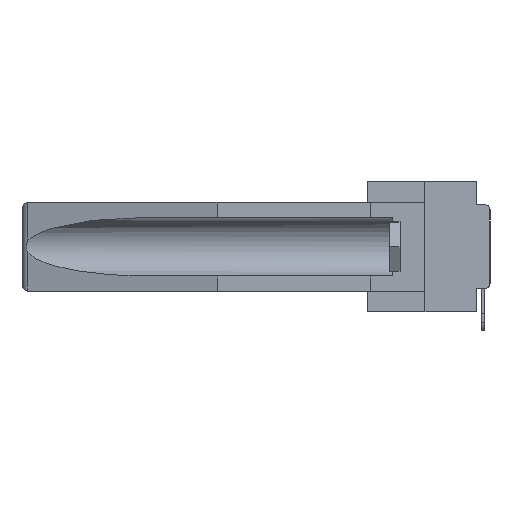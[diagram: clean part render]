
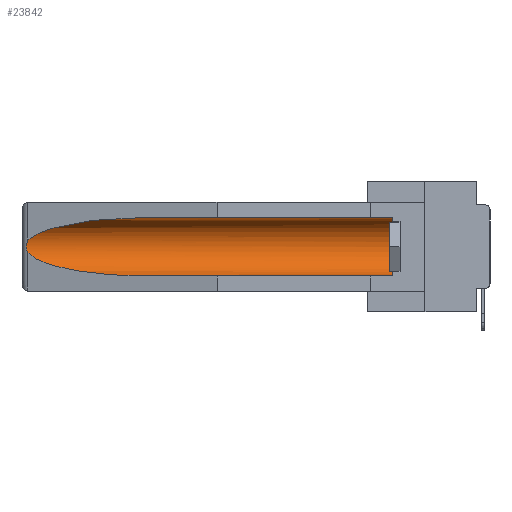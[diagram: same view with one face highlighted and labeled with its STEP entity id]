
A CAD part, left-side view. The second image highlights one B-rep face of the part: STEP entity #23842.
In plain terms, the highlighted cylindrical face has radius 2.857 mm (diameter 5.715 mm), a partial arc.
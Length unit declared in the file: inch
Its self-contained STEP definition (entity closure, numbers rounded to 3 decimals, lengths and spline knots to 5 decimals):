
#638 = ORIENTED_EDGE ( 'NONE', *, *, #23297, .T. ) ;
#746 = CARTESIAN_POINT ( 'NONE',  ( 0.21114, 1.30732, -0.284 ) ) ;
#1210 = EDGE_LOOP ( 'NONE', ( #5220, #638, #20879, #20335, #5488, #31208 ) ) ;
#1312 = DIRECTION ( 'NONE',  ( 0., 0., 1. ) ) ;
#1347 = CARTESIAN_POINT ( 'NONE',  ( 0.2673, 1.5327, -0.16383 ) ) ;
#1713 = EDGE_CURVE ( 'NONE', #22830, #21213, #23108, .T. ) ;
#2689 = EDGE_CURVE ( 'NONE', #28730, #30692, #25787, .T. ) ;
#2841 = VECTOR ( 'NONE', #15297, 39.37008 ) ;
#3569 = DIRECTION ( 'NONE',  ( 0., 1., 0. ) ) ;
#3854 = CYLINDRICAL_SURFACE ( 'NONE', #14177, 0.1125 ) ;
#4030 = CARTESIAN_POINT ( 'NONE',  ( 0.26597, 1.52961, -0.15275 ) ) ;
#4127 = CARTESIAN_POINT ( 'NONE',  ( 0.26537, 1.52718, -0.14972 ) ) ;
#4273 = CARTESIAN_POINT ( 'NONE',  ( 0.21114, 1.30732, -0.059 ) ) ;
#4820 = CARTESIAN_POINT ( 'NONE',  ( 0.155, 1.07973, -0.059 ) ) ;
#4983 = CARTESIAN_POINT ( 'NONE',  ( 0.155, 0.126, -0.284 ) ) ;
#5220 = ORIENTED_EDGE ( 'NONE', *, *, #10701, .T. ) ;
#5488 = ORIENTED_EDGE ( 'NONE', *, *, #2689, .T. ) ;
#5899 = CARTESIAN_POINT ( 'NONE',  ( 0.26537, 1.52718, -0.19328 ) ) ;
#6040 = DIRECTION ( 'NONE',  ( 0., -1., 0. ) ) ;
#6162 = CARTESIAN_POINT ( 'NONE',  ( 0.26537, 1.52718, -0.19328 ) ) ;
#6944 = LINE ( 'NONE', #25351, #17443 ) ;
#8561 = CARTESIAN_POINT ( 'NONE',  ( 0.155, 0.126, -0.059 ) ) ;
#8996 = CARTESIAN_POINT ( 'NONE',  ( 0.26537, 1.52718, -0.19328 ) ) ;
#10531 = CARTESIAN_POINT ( 'NONE',  ( 0.155, 1.07973, -0.284 ) ) ;
#10701 = EDGE_CURVE ( 'NONE', #11907, #15538, #25830, .T. ) ;
#10748 = CARTESIAN_POINT ( 'NONE',  ( 0.26537, 1.52718, -0.14972 ) ) ;
#11437 = CARTESIAN_POINT ( 'NONE',  ( 0.26537, 1.52718, -0.14972 ) ) ;
#11907 = VERTEX_POINT ( 'NONE', #4820 ) ;
#12583 = CARTESIAN_POINT ( 'NONE',  ( 0.155, -0.30754, -0.059 ) ) ;
#12830 = CARTESIAN_POINT ( 'NONE',  ( 0.25451, 1.48313, -0.24835 ) ) ;
#13415 = CARTESIAN_POINT ( 'NONE',  ( 0.2673, 1.53269, -0.17917 ) ) ;
#13831 = CARTESIAN_POINT ( 'NONE',  ( 0.2675, 1.53308, -0.16763 ) ) ;
#13986 = EDGE_CURVE ( 'NONE', #28730, #21213, #6944, .T. ) ;
#14177 = AXIS2_PLACEMENT_3D ( 'NONE', #27528, #3569, #1312 ) ;
#14568 = B_SPLINE_CURVE_WITH_KNOTS ( 'NONE', 3,
 ( #4127, #4030, #23144, #1347, #13831, #18583, #13415, #28303, #25666, #6162 ),
 .UNSPECIFIED., .F., .F.,
 ( 4, 2, 2, 2, 4 ),
 ( 0., 0.00029, 0.00058, 0.00087, 0.00117 ),
 .UNSPECIFIED. ) ;
#15297 = DIRECTION ( 'NONE',  ( 0., 1., 0. ) ) ;
#15314 = LINE ( 'NONE', #12583, #2841 ) ;
#15351 = CARTESIAN_POINT ( 'NONE',  ( 0.155, 1.07973, -0.284 ) ) ;
#15538 = VERTEX_POINT ( 'NONE', #10748 ) ;
#16547 = DIRECTION ( 'NONE',  ( 0., 1., 0. ) ) ;
#17443 = VECTOR ( 'NONE', #16547, 39.37008 ) ;
#18583 = CARTESIAN_POINT ( 'NONE',  ( 0.2675, 1.53308, -0.17534 ) ) ;
#19681 = FACE_OUTER_BOUND ( 'NONE', #1210, .T. ) ;
#20335 = ORIENTED_EDGE ( 'NONE', *, *, #13986, .F. ) ;
#20814 = EDGE_CURVE ( 'NONE', #30692, #11907, #15314, .T. ) ;
#20879 = ORIENTED_EDGE ( 'NONE', *, *, #1713, .T. ) ;
#21150 = CARTESIAN_POINT ( 'NONE',  ( 0.155, 1.07973, -0.059 ) ) ;
#21213 = VERTEX_POINT ( 'NONE', #10531 ) ;
#22830 = VERTEX_POINT ( 'NONE', #8996 ) ;
#23108 =( BOUNDED_CURVE ( )  B_SPLINE_CURVE ( 3, ( #5899, #12830, #746, #15351 ),
 .UNSPECIFIED., .F., .T. ) 
 B_SPLINE_CURVE_WITH_KNOTS ( ( 4, 4 ),
 ( 0.1948, 1.5708 ),
 .UNSPECIFIED. ) 
 CURVE ( )  GEOMETRIC_REPRESENTATION_ITEM ( )  RATIONAL_B_SPLINE_CURVE ( ( 1., 0.848, 0.848, 1. ) ) 
 REPRESENTATION_ITEM ( '' )  );
#23144 = CARTESIAN_POINT ( 'NONE',  ( 0.26654, 1.53092, -0.15636 ) ) ;
#23297 = EDGE_CURVE ( 'NONE', #15538, #22830, #14568, .T. ) ;
#23589 = CARTESIAN_POINT ( 'NONE',  ( 0.25451, 1.48313, -0.09465 ) ) ;
#23842 = ADVANCED_FACE ( 'NONE', ( #19681 ), #3854, .F. ) ;
#25351 = CARTESIAN_POINT ( 'NONE',  ( 0.155, -0.30754, -0.284 ) ) ;
#25666 = CARTESIAN_POINT ( 'NONE',  ( 0.26597, 1.5296, -0.19026 ) ) ;
#25787 = CIRCLE ( 'NONE', #29714, 0.1125 ) ;
#25830 =( BOUNDED_CURVE ( )  B_SPLINE_CURVE ( 3, ( #21150, #4273, #23589, #11437 ),
 .UNSPECIFIED., .F., .F. ) 
 B_SPLINE_CURVE_WITH_KNOTS ( ( 4, 4 ),
 ( 4.71239, 6.08839 ),
 .UNSPECIFIED. ) 
 CURVE ( )  GEOMETRIC_REPRESENTATION_ITEM ( )  RATIONAL_B_SPLINE_CURVE ( ( 1., 0.848, 0.848, 1. ) ) 
 REPRESENTATION_ITEM ( '' )  );
#27528 = CARTESIAN_POINT ( 'NONE',  ( 0.155, -0.30754, -0.1715 ) ) ;
#27985 = DIRECTION ( 'NONE',  ( 0., 0., 1. ) ) ;
#28303 = CARTESIAN_POINT ( 'NONE',  ( 0.26655, 1.53094, -0.18657 ) ) ;
#28730 = VERTEX_POINT ( 'NONE', #4983 ) ;
#29714 = AXIS2_PLACEMENT_3D ( 'NONE', #30109, #6040, #27985 ) ;
#30109 = CARTESIAN_POINT ( 'NONE',  ( 0.155, 0.126, -0.1715 ) ) ;
#30692 = VERTEX_POINT ( 'NONE', #8561 ) ;
#31208 = ORIENTED_EDGE ( 'NONE', *, *, #20814, .T. ) ;
